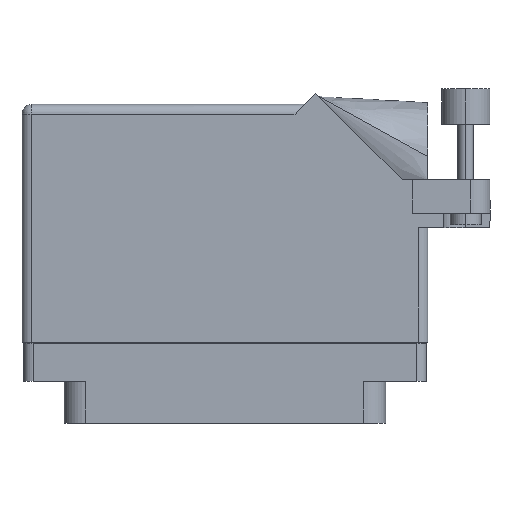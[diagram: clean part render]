
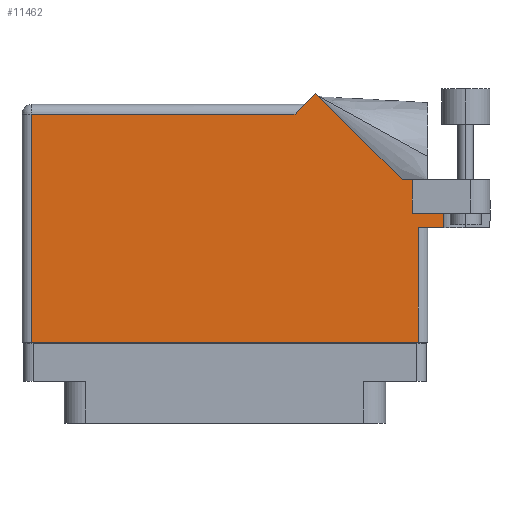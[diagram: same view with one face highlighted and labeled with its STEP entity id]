
A CAD part, front view. The second image highlights one B-rep face of the part: STEP entity #11462.
In plain terms, the highlighted face is planar.
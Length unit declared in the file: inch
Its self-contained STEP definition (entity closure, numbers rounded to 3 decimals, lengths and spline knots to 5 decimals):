
#389 = VERTEX_POINT ( 'NONE', #27605 ) ;
#496 = ORIENTED_EDGE ( 'NONE', *, *, #6274, .F. ) ;
#812 = DIRECTION ( 'NONE',  ( -1., 0., 0. ) ) ;
#855 = VECTOR ( 'NONE', #43730, 39.37008 ) ;
#1726 = VECTOR ( 'NONE', #22607, 39.37008 ) ;
#3495 = VERTEX_POINT ( 'NONE', #39790 ) ;
#3571 = LINE ( 'NONE', #3837, #21602 ) ;
#3815 = VERTEX_POINT ( 'NONE', #41396 ) ;
#3837 = CARTESIAN_POINT ( 'NONE',  ( -1.244, -0.1, 0.455 ) ) ;
#5721 = CARTESIAN_POINT ( 'NONE',  ( -1.244, 1.368, 0.455 ) ) ;
#6274 = EDGE_CURVE ( 'NONE', #3815, #38599, #47538, .T. ) ;
#6358 = LINE ( 'NONE', #33781, #1726 ) ;
#7408 = VERTEX_POINT ( 'NONE', #19911 ) ;
#7545 = DIRECTION ( 'NONE',  ( 0., -1., 0. ) ) ;
#8104 = EDGE_CURVE ( 'NONE', #21566, #33616, #6358, .T. ) ;
#8164 = ORIENTED_EDGE ( 'NONE', *, *, #8104, .T. ) ;
#8419 = EDGE_CURVE ( 'NONE', #389, #41230, #41880, .T. ) ;
#9259 = AXIS2_PLACEMENT_3D ( 'NONE', #12113, #37957, #812 ) ;
#9335 = LINE ( 'NONE', #39233, #32745 ) ;
#9699 = CARTESIAN_POINT ( 'NONE',  ( 1.206, 0.731, 0.455 ) ) ;
#10369 = CARTESIAN_POINT ( 'NONE',  ( 0.513, 1.43, 0.455 ) ) ;
#11462 = ADVANCED_FACE ( 'NONE', ( #18879 ), #19165, .F. ) ;
#12113 = CARTESIAN_POINT ( 'NONE',  ( -1.306, 1.43, 0.455 ) ) ;
#13432 = DIRECTION ( 'NONE',  ( 1., 0., 0. ) ) ;
#13744 = DIRECTION ( 'NONE',  ( 1., 0., 0. ) ) ;
#16522 = CARTESIAN_POINT ( 'NONE',  ( 1.244, -0.1, 0.455 ) ) ;
#17092 = CARTESIAN_POINT ( 'NONE',  ( 1.244, 0.637, 0.455 ) ) ;
#17251 = EDGE_CURVE ( 'NONE', #33616, #35674, #3571, .T. ) ;
#17835 = DIRECTION ( 'NONE',  ( -0.707, 0.707, 0. ) ) ;
#18091 = VECTOR ( 'NONE', #47607, 39.37008 ) ;
#18437 = CARTESIAN_POINT ( 'NONE',  ( 1.4075, 0.637, 0.455 ) ) ;
#18879 = FACE_OUTER_BOUND ( 'NONE', #40007, .T. ) ;
#18934 = EDGE_CURVE ( 'NONE', #41230, #3495, #20112, .T. ) ;
#19165 = PLANE ( 'NONE',  #9259 ) ;
#19454 = CARTESIAN_POINT ( 'NONE',  ( 1.706, 0.944, 0.455 ) ) ;
#19911 = CARTESIAN_POINT ( 'NONE',  ( 0.58371, 1.50071, 0.455 ) ) ;
#20065 = VECTOR ( 'NONE', #13432, 39.37008 ) ;
#20112 = LINE ( 'NONE', #19454, #41772 ) ;
#20652 = CARTESIAN_POINT ( 'NONE',  ( 1.244, 0.637, 0.455 ) ) ;
#21504 = EDGE_CURVE ( 'NONE', #7408, #21566, #27997, .T. ) ;
#21566 = VERTEX_POINT ( 'NONE', #29140 ) ;
#21602 = VECTOR ( 'NONE', #7545, 39.37008 ) ;
#22607 = DIRECTION ( 'NONE',  ( -1., 0., 0. ) ) ;
#23322 = LINE ( 'NONE', #44482, #30354 ) ;
#23789 = ORIENTED_EDGE ( 'NONE', *, *, #35191, .T. ) ;
#24104 = DIRECTION ( 'NONE',  ( 1., 0., 0. ) ) ;
#24744 = VERTEX_POINT ( 'NONE', #20652 ) ;
#25369 = ORIENTED_EDGE ( 'NONE', *, *, #48052, .T. ) ;
#26925 = DIRECTION ( 'NONE',  ( -1., 0., 0. ) ) ;
#27605 = CARTESIAN_POINT ( 'NONE',  ( 1.206, 0.731, 0.455 ) ) ;
#27672 = VERTEX_POINT ( 'NONE', #16522 ) ;
#27997 = LINE ( 'NONE', #10369, #18091 ) ;
#29140 = CARTESIAN_POINT ( 'NONE',  ( 0.451, 1.368, 0.455 ) ) ;
#30315 = CARTESIAN_POINT ( 'NONE',  ( 1.206, 0.944, 0.455 ) ) ;
#30354 = VECTOR ( 'NONE', #17835, 39.37008 ) ;
#31920 = VECTOR ( 'NONE', #47101, 39.37008 ) ;
#32570 = ORIENTED_EDGE ( 'NONE', *, *, #39772, .F. ) ;
#32602 = CARTESIAN_POINT ( 'NONE',  ( -1.244, -0.1, 0.455 ) ) ;
#32745 = VECTOR ( 'NONE', #24104, 39.37008 ) ;
#33469 = LINE ( 'NONE', #47743, #41086 ) ;
#33616 = VERTEX_POINT ( 'NONE', #5721 ) ;
#33781 = CARTESIAN_POINT ( 'NONE',  ( -1.306, 1.368, 0.455 ) ) ;
#35191 = EDGE_CURVE ( 'NONE', #27672, #24744, #39922, .T. ) ;
#35239 = ORIENTED_EDGE ( 'NONE', *, *, #21504, .T. ) ;
#35674 = VERTEX_POINT ( 'NONE', #32602 ) ;
#37373 = EDGE_CURVE ( 'NONE', #35674, #27672, #33469, .T. ) ;
#37576 = ORIENTED_EDGE ( 'NONE', *, *, #18934, .T. ) ;
#37582 = CARTESIAN_POINT ( 'NONE',  ( 1.4075, 1.06177, 0.455 ) ) ;
#37802 = ORIENTED_EDGE ( 'NONE', *, *, #43094, .T. ) ;
#37957 = DIRECTION ( 'NONE',  ( 0., 0., -1. ) ) ;
#38341 = ORIENTED_EDGE ( 'NONE', *, *, #8419, .T. ) ;
#38599 = VERTEX_POINT ( 'NONE', #18437 ) ;
#39233 = CARTESIAN_POINT ( 'NONE',  ( 1.306, 0.637, 0.455 ) ) ;
#39771 = CARTESIAN_POINT ( 'NONE',  ( 1.206, 0.731, 0.455 ) ) ;
#39772 = EDGE_CURVE ( 'NONE', #389, #3815, #47572, .T. ) ;
#39790 = CARTESIAN_POINT ( 'NONE',  ( 1.14042, 0.944, 0.455 ) ) ;
#39922 = LINE ( 'NONE', #17092, #855 ) ;
#40007 = EDGE_LOOP ( 'NONE', ( #44055, #23789, #25369, #496, #32570, #38341, #37576, #37802, #35239, #8164, #40819 ) ) ;
#40819 = ORIENTED_EDGE ( 'NONE', *, *, #17251, .T. ) ;
#41086 = VECTOR ( 'NONE', #13744, 39.37008 ) ;
#41230 = VERTEX_POINT ( 'NONE', #30315 ) ;
#41396 = CARTESIAN_POINT ( 'NONE',  ( 1.4075, 0.731, 0.455 ) ) ;
#41772 = VECTOR ( 'NONE', #26925, 39.37008 ) ;
#41880 = LINE ( 'NONE', #39771, #31920 ) ;
#43094 = EDGE_CURVE ( 'NONE', #3495, #7408, #23322, .T. ) ;
#43730 = DIRECTION ( 'NONE',  ( 0., 1., 0. ) ) ;
#44055 = ORIENTED_EDGE ( 'NONE', *, *, #37373, .T. ) ;
#44482 = CARTESIAN_POINT ( 'NONE',  ( 1.14042, 0.944, 0.455 ) ) ;
#45091 = DIRECTION ( 'NONE',  ( 0., -1., 0. ) ) ;
#46290 = VECTOR ( 'NONE', #45091, 39.37008 ) ;
#47101 = DIRECTION ( 'NONE',  ( 0., 1., 0. ) ) ;
#47538 = LINE ( 'NONE', #37582, #46290 ) ;
#47572 = LINE ( 'NONE', #9699, #20065 ) ;
#47607 = DIRECTION ( 'NONE',  ( -0.707, -0.707, 0. ) ) ;
#47743 = CARTESIAN_POINT ( 'NONE',  ( -1.306, -0.1, 0.455 ) ) ;
#48052 = EDGE_CURVE ( 'NONE', #24744, #38599, #9335, .T. ) ;
